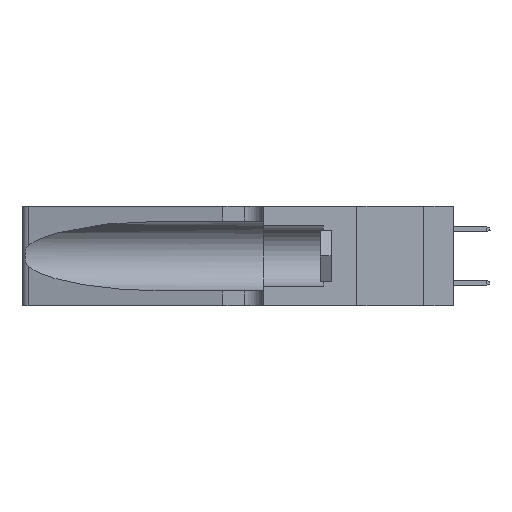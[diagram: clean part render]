
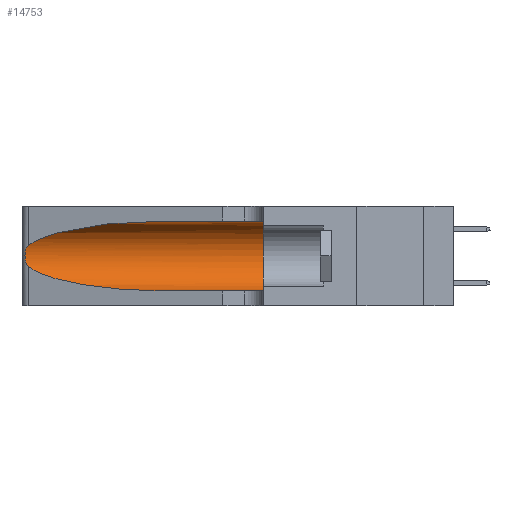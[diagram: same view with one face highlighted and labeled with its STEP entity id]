
A CAD part, left-side view. The second image highlights one B-rep face of the part: STEP entity #14753.
In plain terms, the highlighted cylindrical face has radius 3.308 mm (diameter 6.617 mm), a partial arc.
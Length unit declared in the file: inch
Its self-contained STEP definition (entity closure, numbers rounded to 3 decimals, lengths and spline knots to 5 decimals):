
#845 = LINE ( 'NONE', #28169, #38509 ) ;
#887 = EDGE_CURVE ( 'NONE', #42219, #29240, #14058, .T. ) ;
#942 = VERTEX_POINT ( 'NONE', #15758 ) ;
#2187 =( BOUNDED_CURVE ( )  B_SPLINE_CURVE ( 3, ( #25810, #23182, #36716, #36504 ),
 .UNSPECIFIED., .F., .F. ) 
 B_SPLINE_CURVE_WITH_KNOTS ( ( 4, 4 ),
 ( 3.44316, 4.71239 ),
 .UNSPECIFIED. ) 
 CURVE ( )  GEOMETRIC_REPRESENTATION_ITEM ( )  RATIONAL_B_SPLINE_CURVE ( ( 1., 0.87, 0.87, 1. ) ) 
 REPRESENTATION_ITEM ( '' )  );
#2322 = CARTESIAN_POINT ( 'NONE',  ( 0.26075, 1.23896, 0.178 ) ) ;
#2544 = CARTESIAN_POINT ( 'NONE',  ( 0.2373, 1.15595, 0.28018 ) ) ;
#4421 = CARTESIAN_POINT ( 'NONE',  ( 0.1305, 1.61858, 0.05475 ) ) ;
#4991 = CARTESIAN_POINT ( 'NONE',  ( 0.26017, 1.23833, 0.17102 ) ) ;
#5634 = CARTESIAN_POINT ( 'NONE',  ( 0.25555, 1.22993, 0.14849 ) ) ;
#5795 = AXIS2_PLACEMENT_3D ( 'NONE', #15628, #9085, #38780 ) ;
#8483 = CARTESIAN_POINT ( 'NONE',  ( 0.25487, 1.22718, 0.14631 ) ) ;
#9085 = DIRECTION ( 'NONE',  ( 0., -1., 0. ) ) ;
#9946 = B_SPLINE_CURVE_WITH_KNOTS ( 'NONE', 3,
 ( #14830, #22005, #38402, #35547, #15456, #28574, #42102, #2322, #4991, #18310, #35123, #31839, #5634, #8483 ),
 .UNSPECIFIED., .F., .F.,
 ( 4, 2, 2, 2, 2, 2, 4 ),
 ( 0., 0.00027, 0.00053, 0.00107, 0.0016, 0.00187, 0.00214 ),
 .UNSPECIFIED. ) ;
#10648 = VERTEX_POINT ( 'NONE', #18046 ) ;
#11061 = DIRECTION ( 'NONE',  ( 0., 0., 1. ) ) ;
#13694 = ORIENTED_EDGE ( 'NONE', *, *, #887, .T. ) ;
#14058 = LINE ( 'NONE', #4421, #26262 ) ;
#14210 = DIRECTION ( 'NONE',  ( 0., -1., 0. ) ) ;
#14753 = ADVANCED_FACE ( 'NONE', ( #18897 ), #35289, .F. ) ;
#14830 = CARTESIAN_POINT ( 'NONE',  ( 0.25487, 1.22718, 0.22369 ) ) ;
#15456 = CARTESIAN_POINT ( 'NONE',  ( 0.25854, 1.2359, 0.20912 ) ) ;
#15628 = CARTESIAN_POINT ( 'NONE',  ( 0.1305, 1.61858, 0.185 ) ) ;
#15758 = CARTESIAN_POINT ( 'NONE',  ( 0.25487, 1.22718, 0.14631 ) ) ;
#16242 = AXIS2_PLACEMENT_3D ( 'NONE', #26992, #30490, #11061 ) ;
#16326 = CARTESIAN_POINT ( 'NONE',  ( 0.1305, 0.72297, 0.05475 ) ) ;
#18046 = CARTESIAN_POINT ( 'NONE',  ( 0.1305, 0.72297, 0.31525 ) ) ;
#18310 = CARTESIAN_POINT ( 'NONE',  ( 0.25856, 1.23593, 0.16098 ) ) ;
#18897 = FACE_OUTER_BOUND ( 'NONE', #22329, .T. ) ;
#18914 = ORIENTED_EDGE ( 'NONE', *, *, #33411, .T. ) ;
#19048 = CARTESIAN_POINT ( 'NONE',  ( 0.1305, 0.35, 0.05475 ) ) ;
#19166 = CARTESIAN_POINT ( 'NONE',  ( 0.1305, 0.72297, 0.31525 ) ) ;
#20391 = EDGE_CURVE ( 'NONE', #41688, #942, #9946, .T. ) ;
#22005 = CARTESIAN_POINT ( 'NONE',  ( 0.25555, 1.22994, 0.2215 ) ) ;
#22329 = EDGE_LOOP ( 'NONE', ( #38080, #35856, #18914, #13694, #34268, #32689 ) ) ;
#23182 = CARTESIAN_POINT ( 'NONE',  ( 0.2373, 1.15595, 0.08982 ) ) ;
#23341 = CARTESIAN_POINT ( 'NONE',  ( 0.1305, 0.35, 0.31525 ) ) ;
#25810 = CARTESIAN_POINT ( 'NONE',  ( 0.25487, 1.22718, 0.14631 ) ) ;
#26262 = VECTOR ( 'NONE', #31075, 39.37008 ) ;
#26992 = CARTESIAN_POINT ( 'NONE',  ( 0.1305, 0.35, 0.185 ) ) ;
#28169 = CARTESIAN_POINT ( 'NONE',  ( 0.1305, 1.61858, 0.31525 ) ) ;
#28574 = CARTESIAN_POINT ( 'NONE',  ( 0.26018, 1.23835, 0.19895 ) ) ;
#29008 = CARTESIAN_POINT ( 'NONE',  ( 0.18966, 0.96281, 0.31525 ) ) ;
#29240 = VERTEX_POINT ( 'NONE', #19048 ) ;
#30205 = CIRCLE ( 'NONE', #16242, 0.13025 ) ;
#30364 = EDGE_CURVE ( 'NONE', #32116, #29240, #30205, .T. ) ;
#30490 = DIRECTION ( 'NONE',  ( 0., 1., 0. ) ) ;
#31075 = DIRECTION ( 'NONE',  ( 0., -1., 0. ) ) ;
#31839 = CARTESIAN_POINT ( 'NONE',  ( 0.25639, 1.23186, 0.15144 ) ) ;
#32116 = VERTEX_POINT ( 'NONE', #23341 ) ;
#32689 = ORIENTED_EDGE ( 'NONE', *, *, #39314, .F. ) ;
#32699 = CARTESIAN_POINT ( 'NONE',  ( 0.25487, 1.22718, 0.22369 ) ) ;
#33202 =( BOUNDED_CURVE ( )  B_SPLINE_CURVE ( 3, ( #19166, #29008, #2544, #32699 ),
 .UNSPECIFIED., .F., .F. ) 
 B_SPLINE_CURVE_WITH_KNOTS ( ( 4, 4 ),
 ( 1.5708, 2.84003 ),
 .UNSPECIFIED. ) 
 CURVE ( )  GEOMETRIC_REPRESENTATION_ITEM ( )  RATIONAL_B_SPLINE_CURVE ( ( 1., 0.87, 0.87, 1. ) ) 
 REPRESENTATION_ITEM ( '' )  );
#33411 = EDGE_CURVE ( 'NONE', #942, #42219, #2187, .T. ) ;
#34268 = ORIENTED_EDGE ( 'NONE', *, *, #30364, .F. ) ;
#35123 = CARTESIAN_POINT ( 'NONE',  ( 0.25789, 1.23486, 0.15765 ) ) ;
#35289 = CYLINDRICAL_SURFACE ( 'NONE', #5795, 0.13025 ) ;
#35547 = CARTESIAN_POINT ( 'NONE',  ( 0.25787, 1.23484, 0.2124 ) ) ;
#35856 = ORIENTED_EDGE ( 'NONE', *, *, #20391, .T. ) ;
#36504 = CARTESIAN_POINT ( 'NONE',  ( 0.1305, 0.72297, 0.05475 ) ) ;
#36682 = CARTESIAN_POINT ( 'NONE',  ( 0.25487, 1.22718, 0.22369 ) ) ;
#36716 = CARTESIAN_POINT ( 'NONE',  ( 0.18966, 0.96281, 0.05475 ) ) ;
#38080 = ORIENTED_EDGE ( 'NONE', *, *, #41925, .T. ) ;
#38402 = CARTESIAN_POINT ( 'NONE',  ( 0.25639, 1.23184, 0.21858 ) ) ;
#38509 = VECTOR ( 'NONE', #14210, 39.37008 ) ;
#38780 = DIRECTION ( 'NONE',  ( 0., 0., -1. ) ) ;
#39314 = EDGE_CURVE ( 'NONE', #10648, #32116, #845, .T. ) ;
#41688 = VERTEX_POINT ( 'NONE', #36682 ) ;
#41925 = EDGE_CURVE ( 'NONE', #10648, #41688, #33202, .T. ) ;
#42102 = CARTESIAN_POINT ( 'NONE',  ( 0.26075, 1.23896, 0.19203 ) ) ;
#42219 = VERTEX_POINT ( 'NONE', #16326 ) ;
